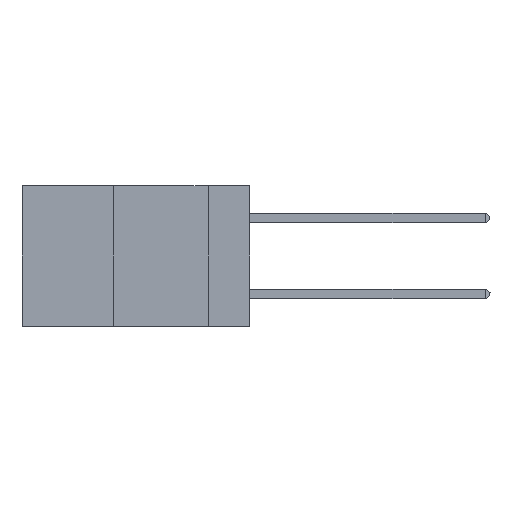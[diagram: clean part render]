
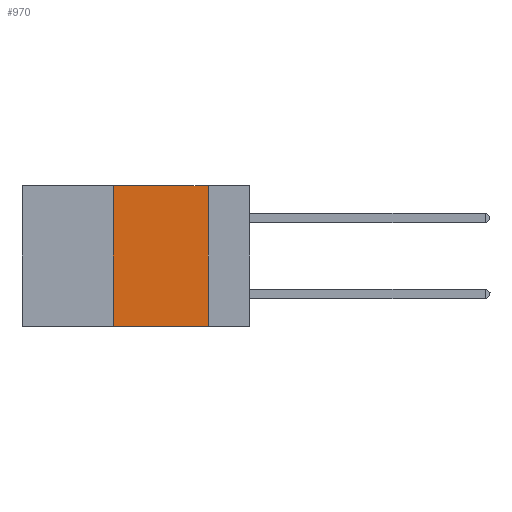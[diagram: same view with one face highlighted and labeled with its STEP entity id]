
A CAD part, left-side view. The second image highlights one B-rep face of the part: STEP entity #970.
In plain terms, the highlighted planar face has unit normal (-1, 0, 0).
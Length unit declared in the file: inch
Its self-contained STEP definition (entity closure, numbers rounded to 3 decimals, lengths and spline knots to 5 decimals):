
#178 = DIRECTION ( 'NONE',  ( 0., 0., -1. ) ) ;
#891 = EDGE_LOOP ( 'NONE', ( #4881, #37533, #9563, #5045 ) ) ;
#928 = VECTOR ( 'NONE', #17674, 39.37008 ) ;
#970 = ADVANCED_FACE ( 'NONE', ( #6967 ), #33567, .F. ) ;
#2082 = CARTESIAN_POINT ( 'NONE',  ( 0., 0.6, 0. ) ) ;
#2448 = LINE ( 'NONE', #22425, #39255 ) ;
#2626 = CARTESIAN_POINT ( 'NONE',  ( 0., 0.36, 0. ) ) ;
#3305 = CARTESIAN_POINT ( 'NONE',  ( 0., 0.36, -0.37 ) ) ;
#4881 = ORIENTED_EDGE ( 'NONE', *, *, #10010, .F. ) ;
#5045 = ORIENTED_EDGE ( 'NONE', *, *, #39742, .T. ) ;
#6967 = FACE_OUTER_BOUND ( 'NONE', #891, .T. ) ;
#9563 = ORIENTED_EDGE ( 'NONE', *, *, #40073, .F. ) ;
#9768 = CARTESIAN_POINT ( 'NONE',  ( 0., 0.11, 0. ) ) ;
#10010 = EDGE_CURVE ( 'NONE', #10032, #16594, #22221, .T. ) ;
#10032 = VERTEX_POINT ( 'NONE', #13689 ) ;
#10894 = VERTEX_POINT ( 'NONE', #3305 ) ;
#13499 = LINE ( 'NONE', #2082, #30091 ) ;
#13600 = CARTESIAN_POINT ( 'NONE',  ( 0., 0.6, 0. ) ) ;
#13689 = CARTESIAN_POINT ( 'NONE',  ( 0., 0.11, 0. ) ) ;
#14839 = CARTESIAN_POINT ( 'NONE',  ( 0., 0.11, -0.37 ) ) ;
#16594 = VERTEX_POINT ( 'NONE', #14839 ) ;
#16958 = DIRECTION ( 'NONE',  ( 1., 0., 0. ) ) ;
#17674 = DIRECTION ( 'NONE',  ( 0., -1., 0. ) ) ;
#19097 = DIRECTION ( 'NONE',  ( 0., -1., 0. ) ) ;
#19847 = VERTEX_POINT ( 'NONE', #2626 ) ;
#21670 = AXIS2_PLACEMENT_3D ( 'NONE', #13600, #16958, #40051 ) ;
#22221 = LINE ( 'NONE', #9768, #27909 ) ;
#22425 = CARTESIAN_POINT ( 'NONE',  ( 0., 0.36, 0. ) ) ;
#24614 = CARTESIAN_POINT ( 'NONE',  ( 0., 0.6, -0.37 ) ) ;
#27909 = VECTOR ( 'NONE', #178, 39.37008 ) ;
#30091 = VECTOR ( 'NONE', #19097, 39.37008 ) ;
#30501 = LINE ( 'NONE', #24614, #928 ) ;
#32545 = EDGE_CURVE ( 'NONE', #19847, #10032, #13499, .T. ) ;
#33567 = PLANE ( 'NONE',  #21670 ) ;
#37533 = ORIENTED_EDGE ( 'NONE', *, *, #32545, .F. ) ;
#39255 = VECTOR ( 'NONE', #39310, 39.37008 ) ;
#39310 = DIRECTION ( 'NONE',  ( 0., 0., 1. ) ) ;
#39742 = EDGE_CURVE ( 'NONE', #10894, #16594, #30501, .T. ) ;
#40051 = DIRECTION ( 'NONE',  ( 0., 0., -1. ) ) ;
#40073 = EDGE_CURVE ( 'NONE', #10894, #19847, #2448, .T. ) ;
